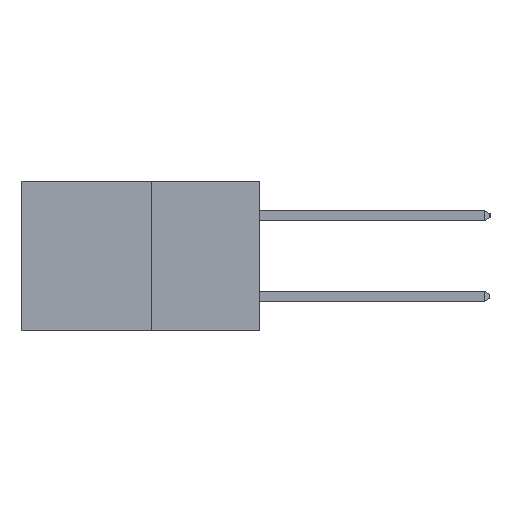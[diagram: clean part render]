
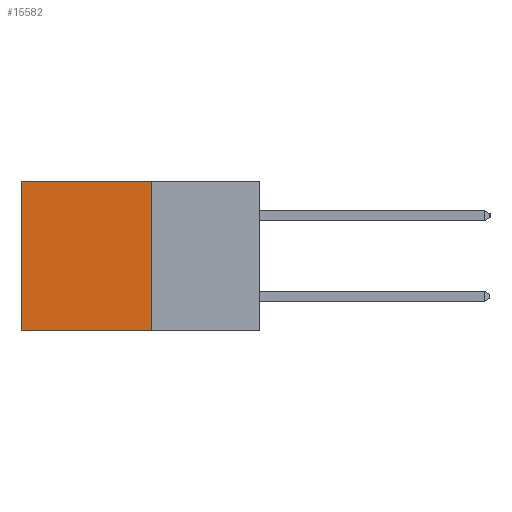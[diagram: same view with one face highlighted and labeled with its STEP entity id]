
A CAD part, left-side view. The second image highlights one B-rep face of the part: STEP entity #15582.
In plain terms, the highlighted planar face has unit normal (-1, 0, 0).
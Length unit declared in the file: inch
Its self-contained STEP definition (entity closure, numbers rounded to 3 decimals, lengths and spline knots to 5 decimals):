
#58 = AXIS2_PLACEMENT_3D ( 'NONE', #15093, #3957, #16970 ) ;
#435 = EDGE_CURVE ( 'NONE', #727, #16343, #536, .T. ) ;
#443 = DIRECTION ( 'NONE',  ( 0., 1., 0. ) ) ;
#536 = LINE ( 'NONE', #2589, #19801 ) ;
#612 = CARTESIAN_POINT ( 'NONE',  ( 0.277, 0.27, -0.37 ) ) ;
#631 = EDGE_LOOP ( 'NONE', ( #18901, #15850, #14195, #7070 ) ) ;
#727 = VERTEX_POINT ( 'NONE', #612 ) ;
#1500 = CARTESIAN_POINT ( 'NONE',  ( 0.277, 0.27, -0.37 ) ) ;
#1625 = EDGE_CURVE ( 'NONE', #17884, #3247, #19452, .T. ) ;
#2589 = CARTESIAN_POINT ( 'NONE',  ( 0.277, 0.27, -0.37 ) ) ;
#3247 = VERTEX_POINT ( 'NONE', #15984 ) ;
#3957 = DIRECTION ( 'NONE',  ( 1., 0., 0. ) ) ;
#4952 = DIRECTION ( 'NONE',  ( 0., 0., -1. ) ) ;
#5532 = LINE ( 'NONE', #17972, #19784 ) ;
#6488 = FACE_OUTER_BOUND ( 'NONE', #631, .T. ) ;
#7070 = ORIENTED_EDGE ( 'NONE', *, *, #1625, .T. ) ;
#9680 = EDGE_CURVE ( 'NONE', #17884, #727, #23805, .T. ) ;
#11418 = PLANE ( 'NONE',  #58 ) ;
#14195 = ORIENTED_EDGE ( 'NONE', *, *, #9680, .F. ) ;
#14498 = VECTOR ( 'NONE', #19620, 39.37008 ) ;
#14652 = VECTOR ( 'NONE', #16415, 39.37008 ) ;
#15093 = CARTESIAN_POINT ( 'NONE',  ( 0.277, 0.27, -0.37 ) ) ;
#15582 = ADVANCED_FACE ( 'NONE', ( #6488 ), #11418, .F. ) ;
#15850 = ORIENTED_EDGE ( 'NONE', *, *, #435, .F. ) ;
#15984 = CARTESIAN_POINT ( 'NONE',  ( 0.277, 0.59, 0. ) ) ;
#16343 = VERTEX_POINT ( 'NONE', #22546 ) ;
#16415 = DIRECTION ( 'NONE',  ( 0., 0., -1. ) ) ;
#16970 = DIRECTION ( 'NONE',  ( 0., 0., -1. ) ) ;
#17250 = EDGE_CURVE ( 'NONE', #3247, #16343, #5532, .T. ) ;
#17884 = VERTEX_POINT ( 'NONE', #21435 ) ;
#17972 = CARTESIAN_POINT ( 'NONE',  ( 0.277, 0.59, -0.37 ) ) ;
#18901 = ORIENTED_EDGE ( 'NONE', *, *, #17250, .T. ) ;
#19452 = LINE ( 'NONE', #19631, #14498 ) ;
#19620 = DIRECTION ( 'NONE',  ( 0., 1., 0. ) ) ;
#19631 = CARTESIAN_POINT ( 'NONE',  ( 0.277, 0.27, 0. ) ) ;
#19784 = VECTOR ( 'NONE', #4952, 39.37008 ) ;
#19801 = VECTOR ( 'NONE', #443, 39.37008 ) ;
#21435 = CARTESIAN_POINT ( 'NONE',  ( 0.277, 0.27, 0. ) ) ;
#22546 = CARTESIAN_POINT ( 'NONE',  ( 0.277, 0.59, -0.37 ) ) ;
#23805 = LINE ( 'NONE', #1500, #14652 ) ;
